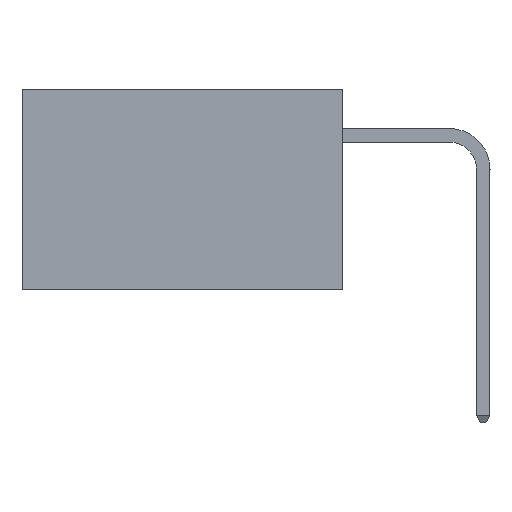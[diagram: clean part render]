
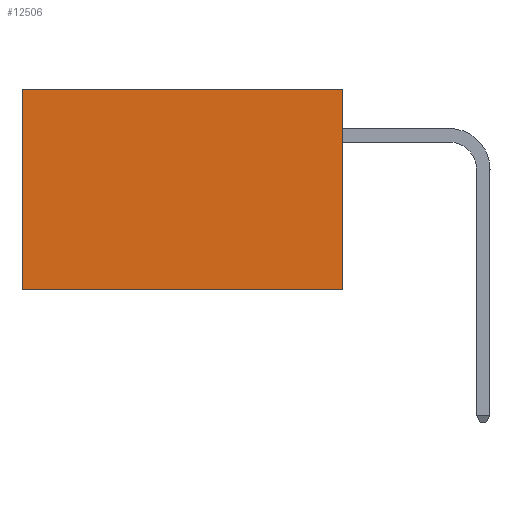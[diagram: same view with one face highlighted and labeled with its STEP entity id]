
A CAD part, left-side view. The second image highlights one B-rep face of the part: STEP entity #12506.
In plain terms, the highlighted planar face has unit normal (-1, 0, 0).
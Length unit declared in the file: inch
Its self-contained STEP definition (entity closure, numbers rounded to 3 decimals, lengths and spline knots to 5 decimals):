
#784 = VECTOR ( 'NONE', #13196, 39.37008 ) ;
#968 = FACE_OUTER_BOUND ( 'NONE', #8347, .T. ) ;
#1185 = CARTESIAN_POINT ( 'NONE',  ( 0.277, 0., -0.37 ) ) ;
#1187 = VERTEX_POINT ( 'NONE', #2518 ) ;
#1719 = DIRECTION ( 'NONE',  ( 0., 1., 0. ) ) ;
#2095 = CARTESIAN_POINT ( 'NONE',  ( 0.277, 0., -0.37 ) ) ;
#2435 = LINE ( 'NONE', #1185, #13113 ) ;
#2436 = CARTESIAN_POINT ( 'NONE',  ( 0.277, 0.59, -0.37 ) ) ;
#2518 = CARTESIAN_POINT ( 'NONE',  ( 0.277, 0.59, 0. ) ) ;
#3061 = CARTESIAN_POINT ( 'NONE',  ( 0.277, 0.59, -0.37 ) ) ;
#3915 = LINE ( 'NONE', #14906, #11112 ) ;
#4275 = EDGE_CURVE ( 'NONE', #7448, #1187, #11611, .T. ) ;
#5103 = DIRECTION ( 'NONE',  ( 0., 0., -1. ) ) ;
#7136 = VERTEX_POINT ( 'NONE', #2436 ) ;
#7177 = EDGE_CURVE ( 'NONE', #13469, #7136, #2435, .T. ) ;
#7418 = ORIENTED_EDGE ( 'NONE', *, *, #7177, .F. ) ;
#7448 = VERTEX_POINT ( 'NONE', #17445 ) ;
#7716 = LINE ( 'NONE', #3061, #784 ) ;
#7835 = CARTESIAN_POINT ( 'NONE',  ( 0.277, 0., -0.37 ) ) ;
#8347 = EDGE_LOOP ( 'NONE', ( #15458, #7418, #17855, #9842 ) ) ;
#9842 = ORIENTED_EDGE ( 'NONE', *, *, #4275, .T. ) ;
#11112 = VECTOR ( 'NONE', #16331, 39.37008 ) ;
#11611 = LINE ( 'NONE', #11753, #14973 ) ;
#11753 = CARTESIAN_POINT ( 'NONE',  ( 0.277, 0., 0. ) ) ;
#12132 = DIRECTION ( 'NONE',  ( 0., 1., 0. ) ) ;
#12506 = ADVANCED_FACE ( 'NONE', ( #968 ), #16476, .F. ) ;
#13113 = VECTOR ( 'NONE', #1719, 39.37008 ) ;
#13196 = DIRECTION ( 'NONE',  ( 0., 0., -1. ) ) ;
#13469 = VERTEX_POINT ( 'NONE', #7835 ) ;
#13719 = DIRECTION ( 'NONE',  ( 1., 0., 0. ) ) ;
#14668 = EDGE_CURVE ( 'NONE', #7448, #13469, #3915, .T. ) ;
#14906 = CARTESIAN_POINT ( 'NONE',  ( 0.277, 0., -0.37 ) ) ;
#14973 = VECTOR ( 'NONE', #12132, 39.37008 ) ;
#15458 = ORIENTED_EDGE ( 'NONE', *, *, #16370, .T. ) ;
#16331 = DIRECTION ( 'NONE',  ( 0., 0., -1. ) ) ;
#16370 = EDGE_CURVE ( 'NONE', #1187, #7136, #7716, .T. ) ;
#16476 = PLANE ( 'NONE',  #17595 ) ;
#17445 = CARTESIAN_POINT ( 'NONE',  ( 0.277, 0., 0. ) ) ;
#17595 = AXIS2_PLACEMENT_3D ( 'NONE', #2095, #13719, #5103 ) ;
#17855 = ORIENTED_EDGE ( 'NONE', *, *, #14668, .F. ) ;
